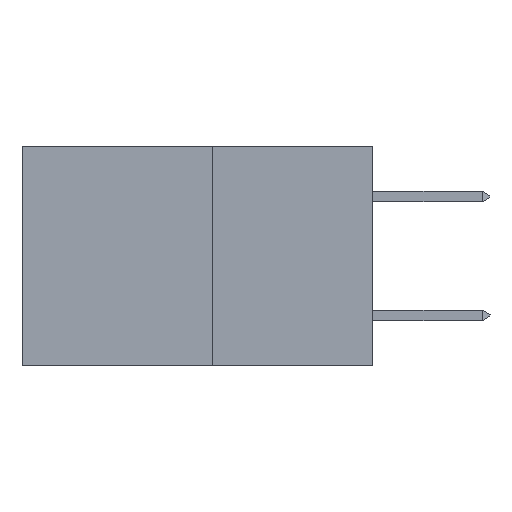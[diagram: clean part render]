
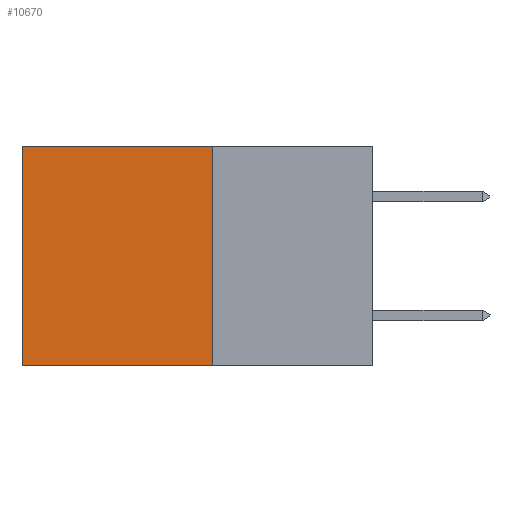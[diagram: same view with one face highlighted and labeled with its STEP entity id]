
A CAD part, left-side view. The second image highlights one B-rep face of the part: STEP entity #10670.
In plain terms, the highlighted planar face has unit normal (-1, 0, 0).
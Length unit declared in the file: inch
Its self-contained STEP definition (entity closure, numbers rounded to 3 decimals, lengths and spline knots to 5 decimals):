
#373 = VERTEX_POINT ( 'NONE', #7406 ) ;
#420 = ORIENTED_EDGE ( 'NONE', *, *, #24221, .T. ) ;
#1751 = DIRECTION ( 'NONE',  ( 0., 0., -1. ) ) ;
#2015 = VECTOR ( 'NONE', #17055, 39.37008 ) ;
#2188 = VECTOR ( 'NONE', #21569, 39.37008 ) ;
#4509 = CARTESIAN_POINT ( 'NONE',  ( 0.277, 0.59, -0.37 ) ) ;
#4578 = VECTOR ( 'NONE', #19095, 39.37008 ) ;
#5811 = ORIENTED_EDGE ( 'NONE', *, *, #15378, .F. ) ;
#6243 = LINE ( 'NONE', #13038, #25676 ) ;
#6868 = ORIENTED_EDGE ( 'NONE', *, *, #32553, .T. ) ;
#7343 = VERTEX_POINT ( 'NONE', #8734 ) ;
#7406 = CARTESIAN_POINT ( 'NONE',  ( 0.277, 0.59, 0. ) ) ;
#8734 = CARTESIAN_POINT ( 'NONE',  ( 0.277, 0.27, -0.37 ) ) ;
#8901 = LINE ( 'NONE', #24013, #2188 ) ;
#10622 = FACE_OUTER_BOUND ( 'NONE', #30559, .T. ) ;
#10670 = ADVANCED_FACE ( 'NONE', ( #10622 ), #11778, .F. ) ;
#11778 = PLANE ( 'NONE',  #26272 ) ;
#13038 = CARTESIAN_POINT ( 'NONE',  ( 0.277, 0.27, 0. ) ) ;
#15378 = EDGE_CURVE ( 'NONE', #7343, #19287, #8901, .T. ) ;
#15569 = DIRECTION ( 'NONE',  ( 0., 1., 0. ) ) ;
#16853 = DIRECTION ( 'NONE',  ( 1., 0., 0. ) ) ;
#17055 = DIRECTION ( 'NONE',  ( 0., 0., -1. ) ) ;
#19095 = DIRECTION ( 'NONE',  ( 0., 0., -1. ) ) ;
#19287 = VERTEX_POINT ( 'NONE', #4509 ) ;
#20134 = ORIENTED_EDGE ( 'NONE', *, *, #23452, .F. ) ;
#21503 = CARTESIAN_POINT ( 'NONE',  ( 0.277, 0.27, -0.37 ) ) ;
#21569 = DIRECTION ( 'NONE',  ( 0., 1., 0. ) ) ;
#22965 = LINE ( 'NONE', #29681, #2015 ) ;
#23452 = EDGE_CURVE ( 'NONE', #30121, #7343, #24768, .T. ) ;
#24013 = CARTESIAN_POINT ( 'NONE',  ( 0.277, 0.27, -0.37 ) ) ;
#24221 = EDGE_CURVE ( 'NONE', #373, #19287, #22965, .T. ) ;
#24768 = LINE ( 'NONE', #21503, #4578 ) ;
#25676 = VECTOR ( 'NONE', #15569, 39.37008 ) ;
#26272 = AXIS2_PLACEMENT_3D ( 'NONE', #26964, #16853, #1751 ) ;
#26964 = CARTESIAN_POINT ( 'NONE',  ( 0.277, 0.27, -0.37 ) ) ;
#29681 = CARTESIAN_POINT ( 'NONE',  ( 0.277, 0.59, -0.37 ) ) ;
#30121 = VERTEX_POINT ( 'NONE', #30199 ) ;
#30199 = CARTESIAN_POINT ( 'NONE',  ( 0.277, 0.27, 0. ) ) ;
#30559 = EDGE_LOOP ( 'NONE', ( #420, #5811, #20134, #6868 ) ) ;
#32553 = EDGE_CURVE ( 'NONE', #30121, #373, #6243, .T. ) ;
